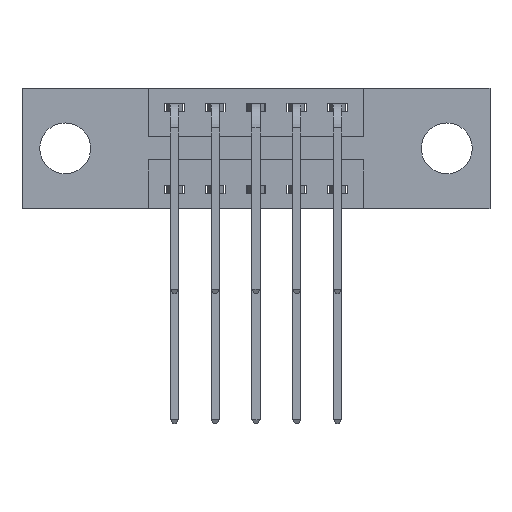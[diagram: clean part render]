
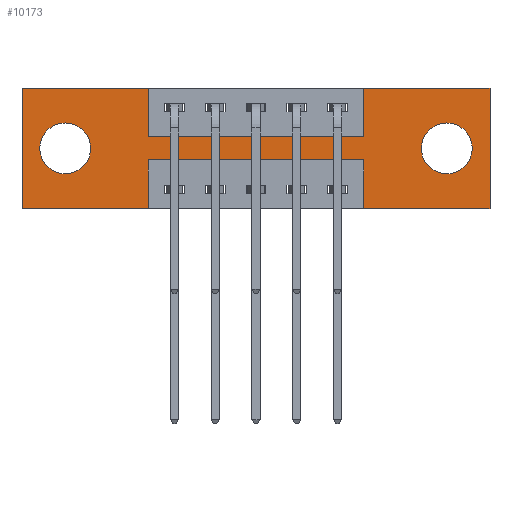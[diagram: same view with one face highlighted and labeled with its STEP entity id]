
A CAD part, front view. The second image highlights one B-rep face of the part: STEP entity #10173.
In plain terms, the highlighted planar face has unit normal (0, -1, 0).
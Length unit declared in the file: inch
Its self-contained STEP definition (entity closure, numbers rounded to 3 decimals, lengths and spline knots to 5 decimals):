
#11 = DIRECTION ( 'NONE',  ( 1., 0., 0. ) ) ;
#47 = VECTOR ( 'NONE', #3135, 39.37008 ) ;
#221 = ORIENTED_EDGE ( 'NONE', *, *, #4868, .T. ) ;
#281 = ORIENTED_EDGE ( 'NONE', *, *, #3251, .F. ) ;
#294 = CARTESIAN_POINT ( 'NONE',  ( 1.3025, 0., -0.185 ) ) ;
#378 = CARTESIAN_POINT ( 'NONE',  ( 1.0475, 0., -0.37 ) ) ;
#399 = VERTEX_POINT ( 'NONE', #8024 ) ;
#415 = CARTESIAN_POINT ( 'NONE',  ( 0.1325, 0., -0.185 ) ) ;
#420 = VERTEX_POINT ( 'NONE', #2604 ) ;
#565 = ORIENTED_EDGE ( 'NONE', *, *, #3173, .F. ) ;
#725 = VERTEX_POINT ( 'NONE', #8005 ) ;
#732 = CARTESIAN_POINT ( 'NONE',  ( 0., 0., -0.37 ) ) ;
#742 = LINE ( 'NONE', #3086, #47 ) ;
#818 = EDGE_CURVE ( 'NONE', #4804, #1182, #3773, .T. ) ;
#945 = CARTESIAN_POINT ( 'NONE',  ( 1.435, 0., 0. ) ) ;
#963 = CARTESIAN_POINT ( 'NONE',  ( 0.3875, 0., -0.22 ) ) ;
#1019 = CARTESIAN_POINT ( 'NONE',  ( 0.3875, 0., 0. ) ) ;
#1178 = VECTOR ( 'NONE', #6549, 39.37008 ) ;
#1182 = VERTEX_POINT ( 'NONE', #7697 ) ;
#1214 = CARTESIAN_POINT ( 'NONE',  ( 1.3025, 0., -0.263 ) ) ;
#1230 = ORIENTED_EDGE ( 'NONE', *, *, #5717, .T. ) ;
#1294 = CARTESIAN_POINT ( 'NONE',  ( 0., 0., 0. ) ) ;
#1313 = VECTOR ( 'NONE', #4501, 39.37008 ) ;
#1598 = LINE ( 'NONE', #4367, #1691 ) ;
#1636 = LINE ( 'NONE', #6833, #6057 ) ;
#1639 = CARTESIAN_POINT ( 'NONE',  ( 1.435, 0., -0.37 ) ) ;
#1649 = CARTESIAN_POINT ( 'NONE',  ( 1.3025, 0., -0.107 ) ) ;
#1691 = VECTOR ( 'NONE', #4847, 39.37008 ) ;
#1885 = LINE ( 'NONE', #945, #5001 ) ;
#2048 = ORIENTED_EDGE ( 'NONE', *, *, #2350, .F. ) ;
#2123 = DIRECTION ( 'NONE',  ( 0., 1., 0. ) ) ;
#2128 = LINE ( 'NONE', #7834, #1178 ) ;
#2190 = EDGE_CURVE ( 'NONE', #1182, #6948, #742, .T. ) ;
#2209 = LINE ( 'NONE', #6908, #6540 ) ;
#2291 = CARTESIAN_POINT ( 'NONE',  ( 1.0475, 0., 0. ) ) ;
#2295 = EDGE_LOOP ( 'NONE', ( #3079, #221 ) ) ;
#2350 = EDGE_CURVE ( 'NONE', #420, #9533, #1885, .T. ) ;
#2448 = EDGE_LOOP ( 'NONE', ( #1230, #4251 ) ) ;
#2452 = ORIENTED_EDGE ( 'NONE', *, *, #4131, .F. ) ;
#2482 = LINE ( 'NONE', #732, #4078 ) ;
#2595 = EDGE_CURVE ( 'NONE', #3009, #8317, #5292, .T. ) ;
#2604 = CARTESIAN_POINT ( 'NONE',  ( 1.435, 0., 0. ) ) ;
#2648 = ORIENTED_EDGE ( 'NONE', *, *, #5861, .F. ) ;
#2736 = LINE ( 'NONE', #378, #5067 ) ;
#2783 = DIRECTION ( 'NONE',  ( 0., 0., -1. ) ) ;
#2791 = VERTEX_POINT ( 'NONE', #3447 ) ;
#2933 = FACE_BOUND ( 'NONE', #2448, .T. ) ;
#2968 = DIRECTION ( 'NONE',  ( 0., 0., 1. ) ) ;
#3009 = VERTEX_POINT ( 'NONE', #6010 ) ;
#3079 = ORIENTED_EDGE ( 'NONE', *, *, #6104, .T. ) ;
#3086 = CARTESIAN_POINT ( 'NONE',  ( 0., 0., 0. ) ) ;
#3135 = DIRECTION ( 'NONE',  ( 1., 0., 0. ) ) ;
#3173 = EDGE_CURVE ( 'NONE', #6948, #3259, #1636, .T. ) ;
#3190 = CIRCLE ( 'NONE', #9112, 0.078 ) ;
#3226 = CIRCLE ( 'NONE', #7738, 0.078 ) ;
#3251 = EDGE_CURVE ( 'NONE', #5602, #3009, #2736, .T. ) ;
#3259 = VERTEX_POINT ( 'NONE', #9285 ) ;
#3447 = CARTESIAN_POINT ( 'NONE',  ( 0.3875, 0., -0.37 ) ) ;
#3509 = DIRECTION ( 'NONE',  ( 0., 0., 1. ) ) ;
#3612 = DIRECTION ( 'NONE',  ( 0., 0., -1. ) ) ;
#3632 = DIRECTION ( 'NONE',  ( 0., 0., 1. ) ) ;
#3708 = AXIS2_PLACEMENT_3D ( 'NONE', #294, #8243, #4923 ) ;
#3773 = LINE ( 'NONE', #1294, #7620 ) ;
#3777 = FACE_OUTER_BOUND ( 'NONE', #9441, .T. ) ;
#3919 = CIRCLE ( 'NONE', #6254, 0.078 ) ;
#4078 = VECTOR ( 'NONE', #5525, 39.37008 ) ;
#4131 = EDGE_CURVE ( 'NONE', #8317, #2791, #2209, .T. ) ;
#4251 = ORIENTED_EDGE ( 'NONE', *, *, #10072, .T. ) ;
#4358 = PLANE ( 'NONE',  #8978 ) ;
#4367 = CARTESIAN_POINT ( 'NONE',  ( 0., 0., 0. ) ) ;
#4486 = VERTEX_POINT ( 'NONE', #1649 ) ;
#4501 = DIRECTION ( 'NONE',  ( -1., 0., 0. ) ) ;
#4673 = ORIENTED_EDGE ( 'NONE', *, *, #2190, .F. ) ;
#4687 = CARTESIAN_POINT ( 'NONE',  ( 0.3875, 0., -0.15 ) ) ;
#4804 = VERTEX_POINT ( 'NONE', #6986 ) ;
#4847 = DIRECTION ( 'NONE',  ( 1., 0., 0. ) ) ;
#4848 = DIRECTION ( 'NONE',  ( 0., 0., 1. ) ) ;
#4868 = EDGE_CURVE ( 'NONE', #5216, #4486, #3190, .T. ) ;
#4923 = DIRECTION ( 'NONE',  ( 0., 0., -1. ) ) ;
#4937 = DIRECTION ( 'NONE',  ( 0., 0., -1. ) ) ;
#5001 = VECTOR ( 'NONE', #4937, 39.37008 ) ;
#5067 = VECTOR ( 'NONE', #3632, 39.37008 ) ;
#5141 = CARTESIAN_POINT ( 'NONE',  ( 0., 0., -0.37 ) ) ;
#5145 = EDGE_CURVE ( 'NONE', #8061, #420, #1598, .T. ) ;
#5216 = VERTEX_POINT ( 'NONE', #1214 ) ;
#5250 = DIRECTION ( 'NONE',  ( 0., 0., -1. ) ) ;
#5292 = LINE ( 'NONE', #8515, #1313 ) ;
#5429 = CARTESIAN_POINT ( 'NONE',  ( 1.0475, 0., 0. ) ) ;
#5460 = LINE ( 'NONE', #4687, #6087 ) ;
#5525 = DIRECTION ( 'NONE',  ( -1., 0., 0. ) ) ;
#5602 = VERTEX_POINT ( 'NONE', #7397 ) ;
#5717 = EDGE_CURVE ( 'NONE', #725, #10030, #3226, .T. ) ;
#5861 = EDGE_CURVE ( 'NONE', #9533, #5602, #2482, .T. ) ;
#6010 = CARTESIAN_POINT ( 'NONE',  ( 1.0475, 0., -0.22 ) ) ;
#6057 = VECTOR ( 'NONE', #6684, 39.37008 ) ;
#6087 = VECTOR ( 'NONE', #11, 39.37008 ) ;
#6104 = EDGE_CURVE ( 'NONE', #4486, #5216, #6387, .T. ) ;
#6129 = DIRECTION ( 'NONE',  ( 0., -1., 0. ) ) ;
#6132 = CARTESIAN_POINT ( 'NONE',  ( 1.3025, 0., -0.185 ) ) ;
#6254 = AXIS2_PLACEMENT_3D ( 'NONE', #8264, #7470, #3509 ) ;
#6358 = EDGE_CURVE ( 'NONE', #399, #8061, #10446, .T. ) ;
#6387 = CIRCLE ( 'NONE', #3708, 0.078 ) ;
#6540 = VECTOR ( 'NONE', #3612, 39.37008 ) ;
#6549 = DIRECTION ( 'NONE',  ( -1., 0., 0. ) ) ;
#6623 = ORIENTED_EDGE ( 'NONE', *, *, #8127, .F. ) ;
#6684 = DIRECTION ( 'NONE',  ( 0., 0., -1. ) ) ;
#6833 = CARTESIAN_POINT ( 'NONE',  ( 0.3875, 0., 0. ) ) ;
#6908 = CARTESIAN_POINT ( 'NONE',  ( 0.3875, 0., -0.37 ) ) ;
#6948 = VERTEX_POINT ( 'NONE', #1019 ) ;
#6986 = CARTESIAN_POINT ( 'NONE',  ( 0., 0., -0.37 ) ) ;
#7177 = EDGE_CURVE ( 'NONE', #2791, #4804, #2128, .T. ) ;
#7182 = ORIENTED_EDGE ( 'NONE', *, *, #7177, .F. ) ;
#7397 = CARTESIAN_POINT ( 'NONE',  ( 1.0475, 0., -0.37 ) ) ;
#7470 = DIRECTION ( 'NONE',  ( 0., 1., 0. ) ) ;
#7565 = FACE_BOUND ( 'NONE', #2295, .T. ) ;
#7620 = VECTOR ( 'NONE', #2968, 39.37008 ) ;
#7697 = CARTESIAN_POINT ( 'NONE',  ( 0., 0., 0. ) ) ;
#7738 = AXIS2_PLACEMENT_3D ( 'NONE', #415, #8516, #10196 ) ;
#7834 = CARTESIAN_POINT ( 'NONE',  ( 0., 0., -0.37 ) ) ;
#8005 = CARTESIAN_POINT ( 'NONE',  ( 0.1325, 0., -0.107 ) ) ;
#8024 = CARTESIAN_POINT ( 'NONE',  ( 1.0475, 0., -0.15 ) ) ;
#8061 = VERTEX_POINT ( 'NONE', #2291 ) ;
#8103 = VECTOR ( 'NONE', #4848, 39.37008 ) ;
#8127 = EDGE_CURVE ( 'NONE', #3259, #399, #5460, .T. ) ;
#8162 = CARTESIAN_POINT ( 'NONE',  ( 0.1325, 0., -0.263 ) ) ;
#8243 = DIRECTION ( 'NONE',  ( 0., 1., 0. ) ) ;
#8255 = ORIENTED_EDGE ( 'NONE', *, *, #5145, .F. ) ;
#8264 = CARTESIAN_POINT ( 'NONE',  ( 0.1325, 0., -0.185 ) ) ;
#8317 = VERTEX_POINT ( 'NONE', #963 ) ;
#8515 = CARTESIAN_POINT ( 'NONE',  ( 0.3875, 0., -0.22 ) ) ;
#8516 = DIRECTION ( 'NONE',  ( 0., 1., 0. ) ) ;
#8876 = ORIENTED_EDGE ( 'NONE', *, *, #818, .F. ) ;
#8978 = AXIS2_PLACEMENT_3D ( 'NONE', #5141, #6129, #2783 ) ;
#9112 = AXIS2_PLACEMENT_3D ( 'NONE', #6132, #2123, #5250 ) ;
#9285 = CARTESIAN_POINT ( 'NONE',  ( 0.3875, 0., -0.15 ) ) ;
#9441 = EDGE_LOOP ( 'NONE', ( #2452, #10043, #281, #2648, #2048, #8255, #9668, #6623, #565, #4673, #8876, #7182 ) ) ;
#9533 = VERTEX_POINT ( 'NONE', #1639 ) ;
#9668 = ORIENTED_EDGE ( 'NONE', *, *, #6358, .F. ) ;
#10030 = VERTEX_POINT ( 'NONE', #8162 ) ;
#10043 = ORIENTED_EDGE ( 'NONE', *, *, #2595, .F. ) ;
#10072 = EDGE_CURVE ( 'NONE', #10030, #725, #3919, .T. ) ;
#10173 = ADVANCED_FACE ( 'NONE', ( #7565, #2933, #3777 ), #4358, .T. ) ;
#10196 = DIRECTION ( 'NONE',  ( 0., 0., 1. ) ) ;
#10446 = LINE ( 'NONE', #5429, #8103 ) ;
